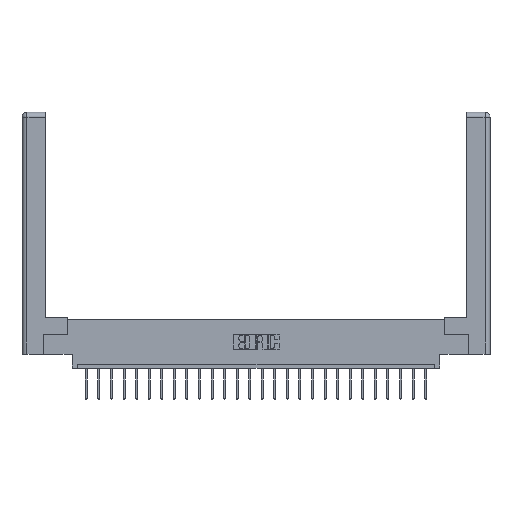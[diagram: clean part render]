
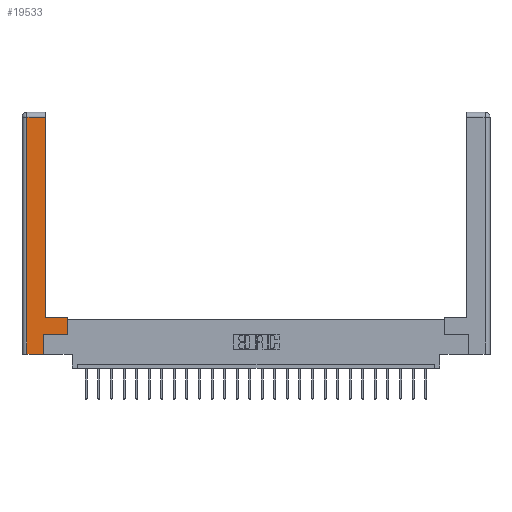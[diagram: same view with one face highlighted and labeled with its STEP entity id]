
A CAD part, top view. The second image highlights one B-rep face of the part: STEP entity #19533.
In plain terms, the highlighted planar face has unit normal (0, 0, 1).
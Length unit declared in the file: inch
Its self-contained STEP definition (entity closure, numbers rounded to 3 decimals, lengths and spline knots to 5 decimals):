
#58 = LINE ( 'NONE', #4309, #4348 ) ;
#132 = VECTOR ( 'NONE', #15769, 39.37008 ) ;
#1189 = VERTEX_POINT ( 'NONE', #9719 ) ;
#2054 = DIRECTION ( 'NONE',  ( 0., 1., 0. ) ) ;
#3506 = LINE ( 'NONE', #23458, #5655 ) ;
#4309 = CARTESIAN_POINT ( 'NONE',  ( 0.295, 3., 0. ) ) ;
#4348 = VECTOR ( 'NONE', #2054, 39.37008 ) ;
#4797 = LINE ( 'NONE', #19626, #20091 ) ;
#5236 = CARTESIAN_POINT ( 'NONE',  ( 0.565, 0.45, 0. ) ) ;
#5249 = EDGE_CURVE ( 'NONE', #1189, #20450, #15040, .T. ) ;
#5437 = EDGE_LOOP ( 'NONE', ( #20921, #15900, #8288, #11011, #12577, #24072, #19558, #7854 ) ) ;
#5655 = VECTOR ( 'NONE', #17569, 39.37008 ) ;
#5857 = DIRECTION ( 'NONE',  ( 0., -1., 0. ) ) ;
#6024 = DIRECTION ( 'NONE',  ( 1., 0., 0. ) ) ;
#6047 = CARTESIAN_POINT ( 'NONE',  ( 0.295, 0.45, 0. ) ) ;
#6364 = CARTESIAN_POINT ( 'NONE',  ( 0.0615, 2.94, 0. ) ) ;
#6746 = VERTEX_POINT ( 'NONE', #14711 ) ;
#6931 = EDGE_CURVE ( 'NONE', #20450, #6746, #4797, .T. ) ;
#7167 = VECTOR ( 'NONE', #7920, 39.37008 ) ;
#7442 = DIRECTION ( 'NONE',  ( 0., 1., 0. ) ) ;
#7854 = ORIENTED_EDGE ( 'NONE', *, *, #16730, .T. ) ;
#7920 = DIRECTION ( 'NONE',  ( -1., 0., 0. ) ) ;
#8288 = ORIENTED_EDGE ( 'NONE', *, *, #5249, .T. ) ;
#8471 = CARTESIAN_POINT ( 'NONE',  ( 0.565, 0.245, 0. ) ) ;
#9453 = VERTEX_POINT ( 'NONE', #10890 ) ;
#9719 = CARTESIAN_POINT ( 'NONE',  ( 0.0615, 2.94, 0. ) ) ;
#10890 = CARTESIAN_POINT ( 'NONE',  ( 0.265, 0.245, 0. ) ) ;
#11011 = ORIENTED_EDGE ( 'NONE', *, *, #6931, .T. ) ;
#11514 = DIRECTION ( 'NONE',  ( -1., 0., 0. ) ) ;
#11684 = CARTESIAN_POINT ( 'NONE',  ( 0.565, 0.45, 0. ) ) ;
#11689 = DIRECTION ( 'NONE',  ( 0., 0., -1. ) ) ;
#11764 = CARTESIAN_POINT ( 'NONE',  ( 0.265, 0.245, 0. ) ) ;
#12577 = ORIENTED_EDGE ( 'NONE', *, *, #24923, .T. ) ;
#12604 = VECTOR ( 'NONE', #5857, 39.37008 ) ;
#13561 = PLANE ( 'NONE',  #13780 ) ;
#13780 = AXIS2_PLACEMENT_3D ( 'NONE', #15362, #11689, #11514 ) ;
#14294 = EDGE_CURVE ( 'NONE', #14373, #22830, #58, .T. ) ;
#14373 = VERTEX_POINT ( 'NONE', #19705 ) ;
#14711 = CARTESIAN_POINT ( 'NONE',  ( 0.265, 0., 0. ) ) ;
#15040 = LINE ( 'NONE', #15962, #12604 ) ;
#15228 = VECTOR ( 'NONE', #7442, 39.37008 ) ;
#15362 = CARTESIAN_POINT ( 'NONE',  ( 0., 0., 0. ) ) ;
#15769 = DIRECTION ( 'NONE',  ( 0., 1., 0. ) ) ;
#15785 = CARTESIAN_POINT ( 'NONE',  ( 0.295, 2.94, 0. ) ) ;
#15900 = ORIENTED_EDGE ( 'NONE', *, *, #21101, .T. ) ;
#15962 = CARTESIAN_POINT ( 'NONE',  ( 0.0615, 0., 0. ) ) ;
#16730 = EDGE_CURVE ( 'NONE', #17752, #14373, #19710, .T. ) ;
#17174 = FACE_OUTER_BOUND ( 'NONE', #5437, .T. ) ;
#17569 = DIRECTION ( 'NONE',  ( 1., 0., 0. ) ) ;
#17639 = LINE ( 'NONE', #5236, #15228 ) ;
#17752 = VERTEX_POINT ( 'NONE', #11684 ) ;
#17985 = VECTOR ( 'NONE', #22089, 39.37008 ) ;
#19533 = ADVANCED_FACE ( 'NONE', ( #17174 ), #13561, .F. ) ;
#19558 = ORIENTED_EDGE ( 'NONE', *, *, #21380, .T. ) ;
#19626 = CARTESIAN_POINT ( 'NONE',  ( 0.265, 0., 0. ) ) ;
#19705 = CARTESIAN_POINT ( 'NONE',  ( 0.295, 0.45, 0. ) ) ;
#19710 = LINE ( 'NONE', #6047, #7167 ) ;
#19805 = CARTESIAN_POINT ( 'NONE',  ( 0.0615, 0., 0. ) ) ;
#20091 = VECTOR ( 'NONE', #6024, 39.37008 ) ;
#20394 = LINE ( 'NONE', #6364, #17985 ) ;
#20450 = VERTEX_POINT ( 'NONE', #19805 ) ;
#20921 = ORIENTED_EDGE ( 'NONE', *, *, #14294, .T. ) ;
#21101 = EDGE_CURVE ( 'NONE', #22830, #1189, #20394, .T. ) ;
#21380 = EDGE_CURVE ( 'NONE', #23772, #17752, #17639, .T. ) ;
#22089 = DIRECTION ( 'NONE',  ( -1., 0., 0. ) ) ;
#22830 = VERTEX_POINT ( 'NONE', #15785 ) ;
#23458 = CARTESIAN_POINT ( 'NONE',  ( 0.565, 0.245, 0. ) ) ;
#23730 = LINE ( 'NONE', #11764, #132 ) ;
#23772 = VERTEX_POINT ( 'NONE', #8471 ) ;
#24072 = ORIENTED_EDGE ( 'NONE', *, *, #24905, .T. ) ;
#24905 = EDGE_CURVE ( 'NONE', #9453, #23772, #3506, .T. ) ;
#24923 = EDGE_CURVE ( 'NONE', #6746, #9453, #23730, .T. ) ;
